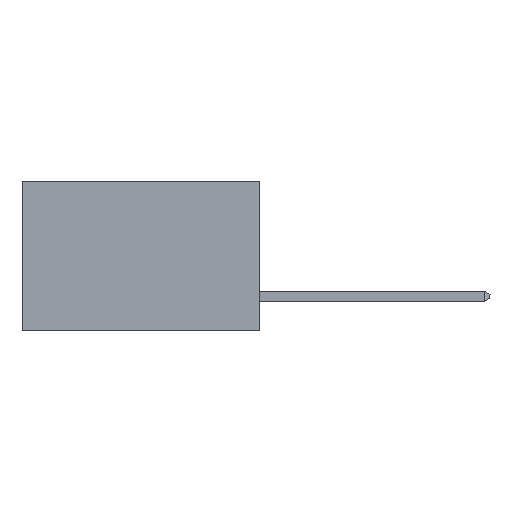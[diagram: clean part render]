
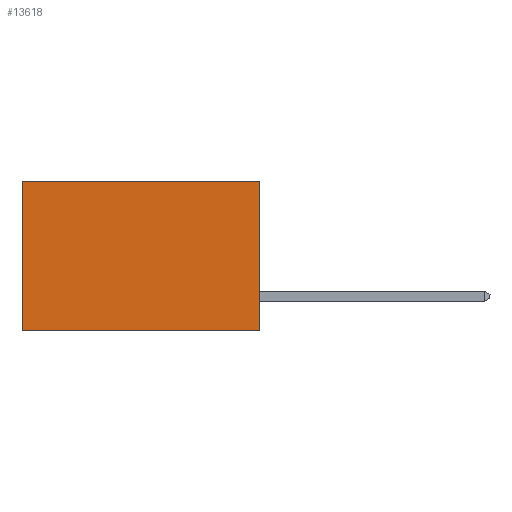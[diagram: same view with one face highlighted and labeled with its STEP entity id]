
A CAD part, left-side view. The second image highlights one B-rep face of the part: STEP entity #13618.
In plain terms, the highlighted planar face has unit normal (-1, 0, 0).
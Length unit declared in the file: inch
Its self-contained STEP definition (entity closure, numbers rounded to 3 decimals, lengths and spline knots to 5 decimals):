
#427 = CARTESIAN_POINT ( 'NONE',  ( 0.277, 0.59, -0.37 ) ) ;
#689 = ORIENTED_EDGE ( 'NONE', *, *, #1302, .T. ) ;
#797 = LINE ( 'NONE', #8101, #6627 ) ;
#1201 = VECTOR ( 'NONE', #3605, 39.37008 ) ;
#1302 = EDGE_CURVE ( 'NONE', #12451, #3810, #14267, .T. ) ;
#1366 = DIRECTION ( 'NONE',  ( 0., 1., 0. ) ) ;
#1420 = CARTESIAN_POINT ( 'NONE',  ( 0.277, 0., 0. ) ) ;
#1450 = EDGE_CURVE ( 'NONE', #5435, #3810, #13131, .T. ) ;
#1476 = EDGE_CURVE ( 'NONE', #4384, #5435, #797, .T. ) ;
#2166 = DIRECTION ( 'NONE',  ( 0., 0., -1. ) ) ;
#3272 = VECTOR ( 'NONE', #2166, 39.37008 ) ;
#3354 = CARTESIAN_POINT ( 'NONE',  ( 0.277, 0., -0.37 ) ) ;
#3605 = DIRECTION ( 'NONE',  ( 0., 1., 0. ) ) ;
#3810 = VERTEX_POINT ( 'NONE', #13649 ) ;
#4384 = VERTEX_POINT ( 'NONE', #10354 ) ;
#4531 = DIRECTION ( 'NONE',  ( 0., 0., -1. ) ) ;
#4558 = CARTESIAN_POINT ( 'NONE',  ( 0.277, 0., -0.37 ) ) ;
#4565 = ORIENTED_EDGE ( 'NONE', *, *, #5074, .T. ) ;
#5074 = EDGE_CURVE ( 'NONE', #4384, #12451, #14461, .T. ) ;
#5435 = VERTEX_POINT ( 'NONE', #9714 ) ;
#6151 = ORIENTED_EDGE ( 'NONE', *, *, #1450, .F. ) ;
#6627 = VECTOR ( 'NONE', #11054, 39.37008 ) ;
#8101 = CARTESIAN_POINT ( 'NONE',  ( 0.277, 0., -0.37 ) ) ;
#9513 = FACE_OUTER_BOUND ( 'NONE', #10834, .T. ) ;
#9714 = CARTESIAN_POINT ( 'NONE',  ( 0.277, 0., -0.37 ) ) ;
#10147 = CARTESIAN_POINT ( 'NONE',  ( 0.277, 0.59, 0. ) ) ;
#10162 = AXIS2_PLACEMENT_3D ( 'NONE', #3354, #11162, #4531 ) ;
#10354 = CARTESIAN_POINT ( 'NONE',  ( 0.277, 0., 0. ) ) ;
#10834 = EDGE_LOOP ( 'NONE', ( #689, #6151, #14144, #4565 ) ) ;
#11054 = DIRECTION ( 'NONE',  ( 0., 0., -1. ) ) ;
#11162 = DIRECTION ( 'NONE',  ( 1., 0., 0. ) ) ;
#12451 = VERTEX_POINT ( 'NONE', #10147 ) ;
#13131 = LINE ( 'NONE', #4558, #1201 ) ;
#13618 = ADVANCED_FACE ( 'NONE', ( #9513 ), #14291, .F. ) ;
#13649 = CARTESIAN_POINT ( 'NONE',  ( 0.277, 0.59, -0.37 ) ) ;
#13816 = VECTOR ( 'NONE', #1366, 39.37008 ) ;
#14144 = ORIENTED_EDGE ( 'NONE', *, *, #1476, .F. ) ;
#14267 = LINE ( 'NONE', #427, #3272 ) ;
#14291 = PLANE ( 'NONE',  #10162 ) ;
#14461 = LINE ( 'NONE', #1420, #13816 ) ;
